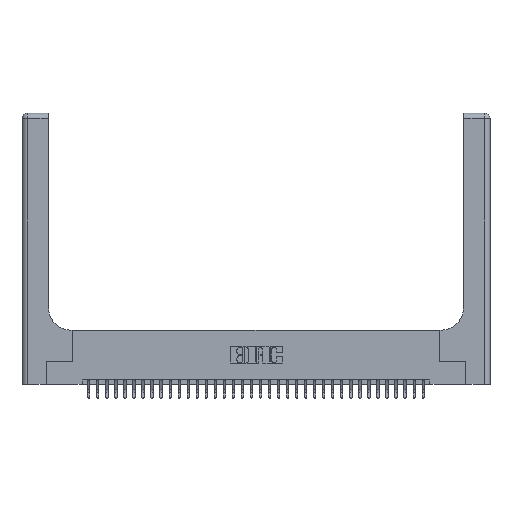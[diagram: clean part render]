
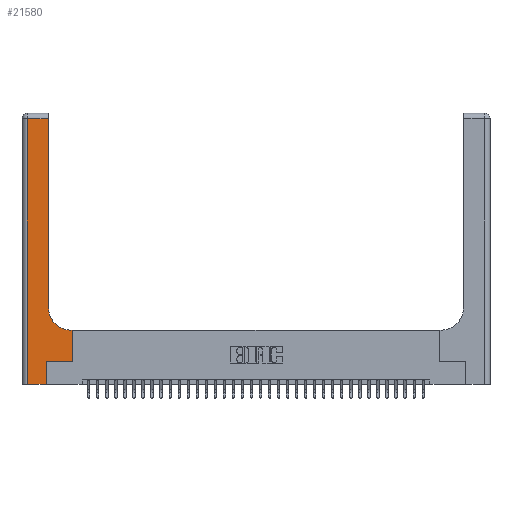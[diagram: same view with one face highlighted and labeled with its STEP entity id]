
A CAD part, top view. The second image highlights one B-rep face of the part: STEP entity #21580.
In plain terms, the highlighted planar face has unit normal (0, 0, 1).
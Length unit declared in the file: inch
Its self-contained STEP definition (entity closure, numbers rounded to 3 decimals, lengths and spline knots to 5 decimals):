
#3 = CARTESIAN_POINT ( 'NONE',  ( 0., 3., 0.37 ) ) ;
#488 = ORIENTED_EDGE ( 'NONE', *, *, #14239, .T. ) ;
#523 = VERTEX_POINT ( 'NONE', #9941 ) ;
#595 = ORIENTED_EDGE ( 'NONE', *, *, #18649, .T. ) ;
#937 = VECTOR ( 'NONE', #15529, 39.37008 ) ;
#1661 = ORIENTED_EDGE ( 'NONE', *, *, #19835, .T. ) ;
#1892 = DIRECTION ( 'NONE',  ( 0., 1., 0. ) ) ;
#2106 = CARTESIAN_POINT ( 'NONE',  ( 0.269, 0., 0.37 ) ) ;
#2344 = VECTOR ( 'NONE', #7382, 39.37008 ) ;
#2419 = VECTOR ( 'NONE', #28566, 39.37008 ) ;
#2475 = FACE_OUTER_BOUND ( 'NONE', #5545, .T. ) ;
#2807 = PLANE ( 'NONE',  #16091 ) ;
#3016 = LINE ( 'NONE', #7968, #6458 ) ;
#3590 = LINE ( 'NONE', #18446, #2344 ) ;
#3969 = EDGE_CURVE ( 'NONE', #11357, #523, #21702, .T. ) ;
#4247 = EDGE_CURVE ( 'NONE', #13968, #11357, #3016, .T. ) ;
#4285 = VERTEX_POINT ( 'NONE', #11572 ) ;
#5545 = EDGE_LOOP ( 'NONE', ( #29344, #30090, #9779, #488, #26512, #595, #12930, #13391, #1661 ) ) ;
#6033 = DIRECTION ( 'NONE',  ( 0., 0., -1. ) ) ;
#6458 = VECTOR ( 'NONE', #8200, 39.37008 ) ;
#7382 = DIRECTION ( 'NONE',  ( -1., 0., 0. ) ) ;
#7968 = CARTESIAN_POINT ( 'NONE',  ( 0.5585, 0.25, 0.37 ) ) ;
#8200 = DIRECTION ( 'NONE',  ( 0., 1., 0. ) ) ;
#8349 = DIRECTION ( 'NONE',  ( -1., 0., 0. ) ) ;
#8512 = DIRECTION ( 'NONE',  ( 1., 0., 0. ) ) ;
#8873 = DIRECTION ( 'NONE',  ( 0., 1., 0. ) ) ;
#9255 = CARTESIAN_POINT ( 'NONE',  ( 0.5585, 0.6, 0.37 ) ) ;
#9779 = ORIENTED_EDGE ( 'NONE', *, *, #32515, .T. ) ;
#9941 = CARTESIAN_POINT ( 'NONE',  ( 0.5415, 0.6, 0.37 ) ) ;
#11248 = EDGE_CURVE ( 'NONE', #4285, #34775, #3590, .T. ) ;
#11357 = VERTEX_POINT ( 'NONE', #9255 ) ;
#11572 = CARTESIAN_POINT ( 'NONE',  ( 0.2915, 2.94, 0.37 ) ) ;
#11820 = VECTOR ( 'NONE', #8512, 39.37008 ) ;
#12930 = ORIENTED_EDGE ( 'NONE', *, *, #4247, .T. ) ;
#13391 = ORIENTED_EDGE ( 'NONE', *, *, #3969, .T. ) ;
#13676 = LINE ( 'NONE', #20620, #2419 ) ;
#13968 = VERTEX_POINT ( 'NONE', #22602 ) ;
#14239 = EDGE_CURVE ( 'NONE', #25107, #19528, #22806, .T. ) ;
#14734 = VECTOR ( 'NONE', #8873, 39.37008 ) ;
#15529 = DIRECTION ( 'NONE',  ( 0., -1., 0. ) ) ;
#15769 = CIRCLE ( 'NONE', #17664, 0.25 ) ;
#16091 = AXIS2_PLACEMENT_3D ( 'NONE', #3, #6033, #8349 ) ;
#17223 = DIRECTION ( 'NONE',  ( 1., 0., 0. ) ) ;
#17664 = AXIS2_PLACEMENT_3D ( 'NONE', #22748, #30825, #17223 ) ;
#17797 = CARTESIAN_POINT ( 'NONE',  ( 0.2915, 0.6, 0.37 ) ) ;
#17904 = CARTESIAN_POINT ( 'NONE',  ( 0.269, 0.25, 0.37 ) ) ;
#18349 = LINE ( 'NONE', #32684, #23926 ) ;
#18446 = CARTESIAN_POINT ( 'NONE',  ( 0., 2.94, 0.37 ) ) ;
#18649 = EDGE_CURVE ( 'NONE', #29064, #13968, #13676, .T. ) ;
#19486 = CARTESIAN_POINT ( 'NONE',  ( 0.2915, 0.85, 0.37 ) ) ;
#19528 = VERTEX_POINT ( 'NONE', #2106 ) ;
#19835 = EDGE_CURVE ( 'NONE', #523, #32761, #15769, .T. ) ;
#20620 = CARTESIAN_POINT ( 'NONE',  ( 0.269, 0.25, 0.37 ) ) ;
#21580 = ADVANCED_FACE ( 'NONE', ( #2475 ), #2807, .F. ) ;
#21702 = LINE ( 'NONE', #17797, #27246 ) ;
#22357 = CARTESIAN_POINT ( 'NONE',  ( 0., 0., 0.37 ) ) ;
#22602 = CARTESIAN_POINT ( 'NONE',  ( 0.5585, 0.25, 0.37 ) ) ;
#22748 = CARTESIAN_POINT ( 'NONE',  ( 0.5415, 0.85, 0.37 ) ) ;
#22806 = LINE ( 'NONE', #22357, #11820 ) ;
#23452 = DIRECTION ( 'NONE',  ( -1., 0., 0. ) ) ;
#23926 = VECTOR ( 'NONE', #1892, 39.37008 ) ;
#25107 = VERTEX_POINT ( 'NONE', #25352 ) ;
#25352 = CARTESIAN_POINT ( 'NONE',  ( 0.06, 0., 0.37 ) ) ;
#26390 = CARTESIAN_POINT ( 'NONE',  ( 0.06, 2.94, 0.37 ) ) ;
#26512 = ORIENTED_EDGE ( 'NONE', *, *, #32078, .T. ) ;
#27246 = VECTOR ( 'NONE', #23452, 39.37008 ) ;
#28566 = DIRECTION ( 'NONE',  ( 1., 0., 0. ) ) ;
#29064 = VERTEX_POINT ( 'NONE', #17904 ) ;
#29344 = ORIENTED_EDGE ( 'NONE', *, *, #35485, .T. ) ;
#29382 = CARTESIAN_POINT ( 'NONE',  ( 0.06, 3., 0.37 ) ) ;
#30090 = ORIENTED_EDGE ( 'NONE', *, *, #11248, .T. ) ;
#30721 = LINE ( 'NONE', #33095, #14734 ) ;
#30825 = DIRECTION ( 'NONE',  ( 0., 0., -1. ) ) ;
#32078 = EDGE_CURVE ( 'NONE', #19528, #29064, #18349, .T. ) ;
#32515 = EDGE_CURVE ( 'NONE', #34775, #25107, #34644, .T. ) ;
#32684 = CARTESIAN_POINT ( 'NONE',  ( 0.269, 0., 0.37 ) ) ;
#32761 = VERTEX_POINT ( 'NONE', #19486 ) ;
#33095 = CARTESIAN_POINT ( 'NONE',  ( 0.2915, 3., 0.37 ) ) ;
#34644 = LINE ( 'NONE', #29382, #937 ) ;
#34775 = VERTEX_POINT ( 'NONE', #26390 ) ;
#35485 = EDGE_CURVE ( 'NONE', #32761, #4285, #30721, .T. ) ;
